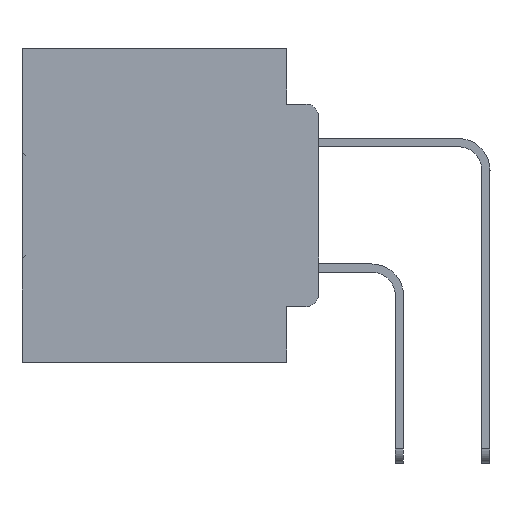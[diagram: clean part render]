
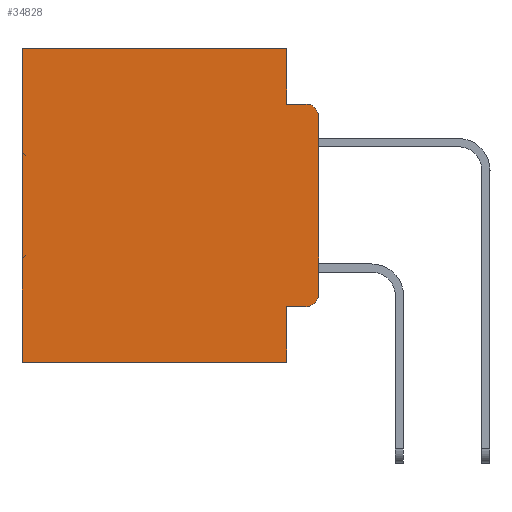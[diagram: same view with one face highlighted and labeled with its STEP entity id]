
A CAD part, left-side view. The second image highlights one B-rep face of the part: STEP entity #34828.
In plain terms, the highlighted planar face has unit normal (-1, 0, 0).
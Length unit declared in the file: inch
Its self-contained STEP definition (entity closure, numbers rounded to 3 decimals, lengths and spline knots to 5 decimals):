
#102 = CARTESIAN_POINT ( 'NONE',  ( 0.298, 0., 0. ) ) ;
#230 = ORIENTED_EDGE ( 'NONE', *, *, #18562, .T. ) ;
#1471 = VECTOR ( 'NONE', #22841, 39.37008 ) ;
#1640 = LINE ( 'NONE', #28259, #29256 ) ;
#1874 = CARTESIAN_POINT ( 'NONE',  ( 0.298, 0.051, 0. ) ) ;
#2153 = LINE ( 'NONE', #30052, #4782 ) ;
#2441 = ORIENTED_EDGE ( 'NONE', *, *, #16683, .T. ) ;
#2553 = LINE ( 'NONE', #1874, #13100 ) ;
#2777 = EDGE_LOOP ( 'NONE', ( #19615, #26421, #10515, #13078, #24581, #18003, #8939, #8029, #230, #2441 ) ) ;
#4087 = VECTOR ( 'NONE', #22199, 39.37008 ) ;
#4218 = CIRCLE ( 'NONE', #25749, 0.02 ) ;
#4500 = EDGE_CURVE ( 'NONE', #29840, #32331, #2153, .T. ) ;
#4540 = VERTEX_POINT ( 'NONE', #16098 ) ;
#4549 = CARTESIAN_POINT ( 'NONE',  ( 0.298, 0.051, -0.4115 ) ) ;
#4782 = VECTOR ( 'NONE', #33695, 39.37008 ) ;
#4944 = VECTOR ( 'NONE', #6754, 39.37008 ) ;
#6748 = DIRECTION ( 'NONE',  ( 0., 0., -1. ) ) ;
#6754 = DIRECTION ( 'NONE',  ( 0., -1., 0. ) ) ;
#6780 = CARTESIAN_POINT ( 'NONE',  ( 0.298, 0., -0.1085 ) ) ;
#7254 = LINE ( 'NONE', #12873, #12956 ) ;
#7425 = CARTESIAN_POINT ( 'NONE',  ( 0.298, 0.02, -0.4115 ) ) ;
#8029 = ORIENTED_EDGE ( 'NONE', *, *, #35275, .F. ) ;
#8939 = ORIENTED_EDGE ( 'NONE', *, *, #20752, .F. ) ;
#9698 = DIRECTION ( 'NONE',  ( -1., 0., 0. ) ) ;
#10033 = FACE_OUTER_BOUND ( 'NONE', #2777, .T. ) ;
#10052 = VERTEX_POINT ( 'NONE', #6780 ) ;
#10515 = ORIENTED_EDGE ( 'NONE', *, *, #15829, .F. ) ;
#11528 = DIRECTION ( 'NONE',  ( 0., 0., -1. ) ) ;
#12720 = VERTEX_POINT ( 'NONE', #4549 ) ;
#12873 = CARTESIAN_POINT ( 'NONE',  ( 0.298, 0.051, 0. ) ) ;
#12956 = VECTOR ( 'NONE', #13250, 39.37008 ) ;
#13078 = ORIENTED_EDGE ( 'NONE', *, *, #16789, .F. ) ;
#13100 = VECTOR ( 'NONE', #32985, 39.37008 ) ;
#13250 = DIRECTION ( 'NONE',  ( 0., 0., -1. ) ) ;
#14744 = CIRCLE ( 'NONE', #27640, 0.02 ) ;
#15112 = LINE ( 'NONE', #102, #23434 ) ;
#15829 = EDGE_CURVE ( 'NONE', #26295, #17612, #1640, .T. ) ;
#15836 = CARTESIAN_POINT ( 'NONE',  ( 0.298, 0.473, -0.5 ) ) ;
#16098 = CARTESIAN_POINT ( 'NONE',  ( 0.298, 0.051, -0.5 ) ) ;
#16350 = LINE ( 'NONE', #30393, #4087 ) ;
#16522 = EDGE_CURVE ( 'NONE', #10052, #17612, #14744, .T. ) ;
#16683 = EDGE_CURVE ( 'NONE', #18015, #34362, #4218, .T. ) ;
#16789 = EDGE_CURVE ( 'NONE', #29840, #26295, #7254, .T. ) ;
#17007 = CARTESIAN_POINT ( 'NONE',  ( 0.298, 0.02, -0.0885 ) ) ;
#17612 = VERTEX_POINT ( 'NONE', #17007 ) ;
#18003 = ORIENTED_EDGE ( 'NONE', *, *, #27667, .T. ) ;
#18015 = VERTEX_POINT ( 'NONE', #7425 ) ;
#18373 = CARTESIAN_POINT ( 'NONE',  ( 0.298, 0.051, -0.0885 ) ) ;
#18562 = EDGE_CURVE ( 'NONE', #12720, #18015, #22491, .T. ) ;
#19044 = CARTESIAN_POINT ( 'NONE',  ( 0.298, 0.473, 0. ) ) ;
#19541 = DIRECTION ( 'NONE',  ( 0., 0., -1. ) ) ;
#19615 = ORIENTED_EDGE ( 'NONE', *, *, #26582, .F. ) ;
#20003 = DIRECTION ( 'NONE',  ( 1., 0., 0. ) ) ;
#20127 = DIRECTION ( 'NONE',  ( -1., 0., 0. ) ) ;
#20752 = EDGE_CURVE ( 'NONE', #4540, #29728, #30399, .T. ) ;
#22199 = DIRECTION ( 'NONE',  ( 0., 0., -1. ) ) ;
#22491 = LINE ( 'NONE', #34691, #4944 ) ;
#22841 = DIRECTION ( 'NONE',  ( 0., 1., 0. ) ) ;
#23434 = VECTOR ( 'NONE', #33982, 39.37008 ) ;
#24581 = ORIENTED_EDGE ( 'NONE', *, *, #4500, .T. ) ;
#25400 = CARTESIAN_POINT ( 'NONE',  ( 0.298, 0., 0. ) ) ;
#25533 = CARTESIAN_POINT ( 'NONE',  ( 0.298, 0., -0.5 ) ) ;
#25563 = CARTESIAN_POINT ( 'NONE',  ( 0.298, 0., -0.3915 ) ) ;
#25749 = AXIS2_PLACEMENT_3D ( 'NONE', #34686, #9698, #6748 ) ;
#26003 = CARTESIAN_POINT ( 'NONE',  ( 0.298, 0.02, -0.1085 ) ) ;
#26295 = VERTEX_POINT ( 'NONE', #18373 ) ;
#26421 = ORIENTED_EDGE ( 'NONE', *, *, #16522, .T. ) ;
#26582 = EDGE_CURVE ( 'NONE', #10052, #34362, #15112, .T. ) ;
#27640 = AXIS2_PLACEMENT_3D ( 'NONE', #26003, #20127, #11528 ) ;
#27667 = EDGE_CURVE ( 'NONE', #32331, #29728, #16350, .T. ) ;
#28259 = CARTESIAN_POINT ( 'NONE',  ( 0.298, 0.051, -0.0885 ) ) ;
#29256 = VECTOR ( 'NONE', #30948, 39.37008 ) ;
#29545 = CARTESIAN_POINT ( 'NONE',  ( 0.298, 0.051, 0. ) ) ;
#29728 = VERTEX_POINT ( 'NONE', #15836 ) ;
#29840 = VERTEX_POINT ( 'NONE', #29545 ) ;
#30052 = CARTESIAN_POINT ( 'NONE',  ( 0.298, 0., 0. ) ) ;
#30393 = CARTESIAN_POINT ( 'NONE',  ( 0.298, 0.473, 0. ) ) ;
#30399 = LINE ( 'NONE', #25533, #1471 ) ;
#30948 = DIRECTION ( 'NONE',  ( 0., -1., 0. ) ) ;
#31150 = PLANE ( 'NONE',  #32761 ) ;
#32331 = VERTEX_POINT ( 'NONE', #19044 ) ;
#32761 = AXIS2_PLACEMENT_3D ( 'NONE', #25400, #20003, #19541 ) ;
#32985 = DIRECTION ( 'NONE',  ( 0., 0., -1. ) ) ;
#33695 = DIRECTION ( 'NONE',  ( 0., 1., 0. ) ) ;
#33982 = DIRECTION ( 'NONE',  ( 0., 0., -1. ) ) ;
#34362 = VERTEX_POINT ( 'NONE', #25563 ) ;
#34686 = CARTESIAN_POINT ( 'NONE',  ( 0.298, 0.02, -0.3915 ) ) ;
#34691 = CARTESIAN_POINT ( 'NONE',  ( 0.298, 0.051, -0.4115 ) ) ;
#34828 = ADVANCED_FACE ( 'NONE', ( #10033 ), #31150, .F. ) ;
#35275 = EDGE_CURVE ( 'NONE', #12720, #4540, #2553, .T. ) ;
